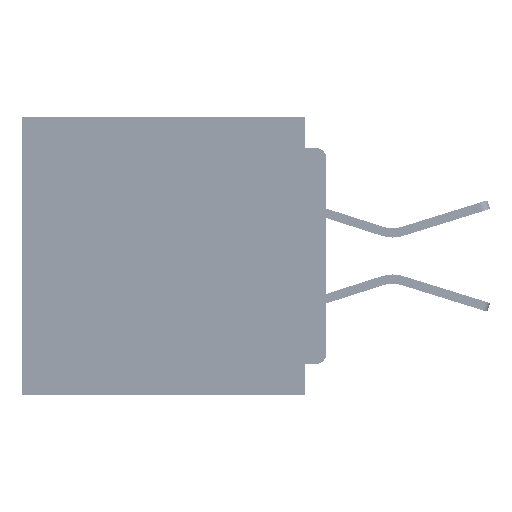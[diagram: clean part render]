
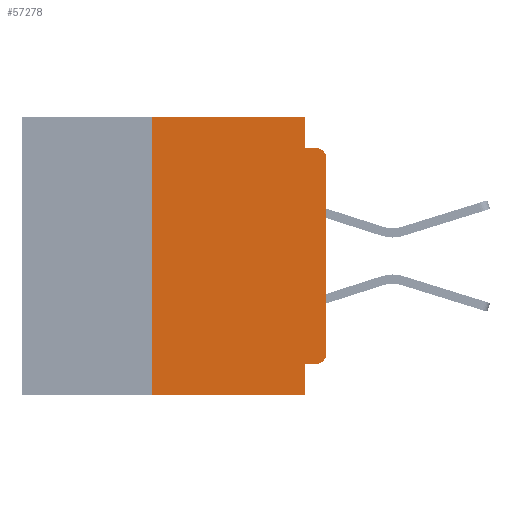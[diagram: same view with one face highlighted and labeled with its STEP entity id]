
A CAD part, left-side view. The second image highlights one B-rep face of the part: STEP entity #57278.
In plain terms, the highlighted planar face has unit normal (-1, 0, 0).
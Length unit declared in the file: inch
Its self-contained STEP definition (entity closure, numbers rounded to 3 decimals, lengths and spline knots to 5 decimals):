
#643 = ORIENTED_EDGE ( 'NONE', *, *, #56176, .F. ) ;
#1257 = AXIS2_PLACEMENT_3D ( 'NONE', #48206, #16533, #53520 ) ;
#1712 = EDGE_CURVE ( 'NONE', #65344, #35225, #22927, .T. ) ;
#2363 = VECTOR ( 'NONE', #48144, 39.37008 ) ;
#2925 = VERTEX_POINT ( 'NONE', #28663 ) ;
#3128 = CARTESIAN_POINT ( 'NONE',  ( 0., 0., -0.045 ) ) ;
#3157 = CIRCLE ( 'NONE', #41771, 0.015 ) ;
#3234 = CARTESIAN_POINT ( 'NONE',  ( 0., 0.015, -0.355 ) ) ;
#4686 = LINE ( 'NONE', #14722, #60964 ) ;
#6895 = DIRECTION ( 'NONE',  ( 0., -1., 0. ) ) ;
#7356 = LINE ( 'NONE', #35289, #61928 ) ;
#8021 = DIRECTION ( 'NONE',  ( 0., 0., 1. ) ) ;
#8457 = ORIENTED_EDGE ( 'NONE', *, *, #18073, .T. ) ;
#8609 = ORIENTED_EDGE ( 'NONE', *, *, #56729, .F. ) ;
#11054 = EDGE_CURVE ( 'NONE', #37208, #35153, #3157, .T. ) ;
#11843 = VECTOR ( 'NONE', #43680, 39.37008 ) ;
#12291 = DIRECTION ( 'NONE',  ( 0., 0., -1. ) ) ;
#12355 = DIRECTION ( 'NONE',  ( -1., 0., 0. ) ) ;
#12444 = CARTESIAN_POINT ( 'NONE',  ( 0., 0.015, -0.06 ) ) ;
#12999 = ORIENTED_EDGE ( 'NONE', *, *, #53912, .F. ) ;
#13603 = CARTESIAN_POINT ( 'NONE',  ( 0., 0.031, -0.4 ) ) ;
#14722 = CARTESIAN_POINT ( 'NONE',  ( 0., 0., -0.355 ) ) ;
#15848 = LINE ( 'NONE', #42786, #17516 ) ;
#16228 = ORIENTED_EDGE ( 'NONE', *, *, #58459, .T. ) ;
#16316 = VERTEX_POINT ( 'NONE', #13603 ) ;
#16397 = DIRECTION ( 'NONE',  ( 0., -1., 0. ) ) ;
#16533 = DIRECTION ( 'NONE',  ( 1., 0., 0. ) ) ;
#17516 = VECTOR ( 'NONE', #16397, 39.37008 ) ;
#18073 = EDGE_CURVE ( 'NONE', #35153, #65344, #24891, .T. ) ;
#20800 = DIRECTION ( 'NONE',  ( -1., 0., 0. ) ) ;
#20991 = EDGE_CURVE ( 'NONE', #27909, #35225, #48435, .T. ) ;
#22014 = VERTEX_POINT ( 'NONE', #34155 ) ;
#22927 = CIRCLE ( 'NONE', #64761, 0.015 ) ;
#23012 = CARTESIAN_POINT ( 'NONE',  ( 0., 0.031, 0. ) ) ;
#23537 = EDGE_CURVE ( 'NONE', #37208, #55369, #4686, .T. ) ;
#24891 = LINE ( 'NONE', #55711, #49696 ) ;
#26288 = CARTESIAN_POINT ( 'NONE',  ( 0., 0.031, -0.045 ) ) ;
#26915 = CARTESIAN_POINT ( 'NONE',  ( 0., 0.031, -0.4 ) ) ;
#27717 = CARTESIAN_POINT ( 'NONE',  ( 0., 0.25, -0.4 ) ) ;
#27869 = ORIENTED_EDGE ( 'NONE', *, *, #23537, .F. ) ;
#27909 = VERTEX_POINT ( 'NONE', #26288 ) ;
#28663 = CARTESIAN_POINT ( 'NONE',  ( 0., 0.25, -0.4 ) ) ;
#32731 = VECTOR ( 'NONE', #61667, 39.37008 ) ;
#34155 = CARTESIAN_POINT ( 'NONE',  ( 0., 0.25, 0. ) ) ;
#35068 = CARTESIAN_POINT ( 'NONE',  ( 0., 0., -0.34 ) ) ;
#35153 = VERTEX_POINT ( 'NONE', #35068 ) ;
#35225 = VERTEX_POINT ( 'NONE', #62008 ) ;
#35289 = CARTESIAN_POINT ( 'NONE',  ( 0., 0.031, 0. ) ) ;
#35664 = ORIENTED_EDGE ( 'NONE', *, *, #20991, .F. ) ;
#37208 = VERTEX_POINT ( 'NONE', #3234 ) ;
#41677 = LINE ( 'NONE', #27717, #11843 ) ;
#41771 = AXIS2_PLACEMENT_3D ( 'NONE', #52461, #20800, #57744 ) ;
#42786 = CARTESIAN_POINT ( 'NONE',  ( 0., 0.437, -0.4 ) ) ;
#42915 = PLANE ( 'NONE',  #1257 ) ;
#43075 = LINE ( 'NONE', #26915, #2363 ) ;
#43680 = DIRECTION ( 'NONE',  ( 0., 0., 1. ) ) ;
#44746 = ORIENTED_EDGE ( 'NONE', *, *, #11054, .T. ) ;
#45253 = ORIENTED_EDGE ( 'NONE', *, *, #1712, .T. ) ;
#45923 = DIRECTION ( 'NONE',  ( 0., 0., -1. ) ) ;
#48144 = DIRECTION ( 'NONE',  ( 0., 0., -1. ) ) ;
#48206 = CARTESIAN_POINT ( 'NONE',  ( 0., 0.437, 0. ) ) ;
#48435 = LINE ( 'NONE', #3128, #32731 ) ;
#49696 = VECTOR ( 'NONE', #8021, 39.37008 ) ;
#50216 = CARTESIAN_POINT ( 'NONE',  ( 0., 0., -0.06 ) ) ;
#51744 = DIRECTION ( 'NONE',  ( 0., 1., 0. ) ) ;
#52461 = CARTESIAN_POINT ( 'NONE',  ( 0., 0.015, -0.34 ) ) ;
#52929 = EDGE_CURVE ( 'NONE', #55369, #16316, #43075, .T. ) ;
#53520 = DIRECTION ( 'NONE',  ( 0., 0., -1. ) ) ;
#53912 = EDGE_CURVE ( 'NONE', #63647, #27909, #7356, .T. ) ;
#54583 = CARTESIAN_POINT ( 'NONE',  ( 0., 0.437, 0. ) ) ;
#55369 = VERTEX_POINT ( 'NONE', #68051 ) ;
#55711 = CARTESIAN_POINT ( 'NONE',  ( 0., 0., 0. ) ) ;
#56176 = EDGE_CURVE ( 'NONE', #22014, #63647, #65625, .T. ) ;
#56729 = EDGE_CURVE ( 'NONE', #2925, #22014, #41677, .T. ) ;
#57278 = ADVANCED_FACE ( 'NONE', ( #59670 ), #42915, .F. ) ;
#57744 = DIRECTION ( 'NONE',  ( 0., 0., -1. ) ) ;
#58459 = EDGE_CURVE ( 'NONE', #2925, #16316, #15848, .T. ) ;
#59670 = FACE_OUTER_BOUND ( 'NONE', #60410, .T. ) ;
#60410 = EDGE_LOOP ( 'NONE', ( #8457, #45253, #35664, #12999, #643, #8609, #16228, #62188, #27869, #44746 ) ) ;
#60659 = VECTOR ( 'NONE', #6895, 39.37008 ) ;
#60964 = VECTOR ( 'NONE', #51744, 39.37008 ) ;
#61667 = DIRECTION ( 'NONE',  ( 0., -1., 0. ) ) ;
#61928 = VECTOR ( 'NONE', #45923, 39.37008 ) ;
#62008 = CARTESIAN_POINT ( 'NONE',  ( 0., 0.015, -0.045 ) ) ;
#62188 = ORIENTED_EDGE ( 'NONE', *, *, #52929, .F. ) ;
#63647 = VERTEX_POINT ( 'NONE', #23012 ) ;
#64761 = AXIS2_PLACEMENT_3D ( 'NONE', #12444, #12355, #12291 ) ;
#65344 = VERTEX_POINT ( 'NONE', #50216 ) ;
#65625 = LINE ( 'NONE', #54583, #60659 ) ;
#68051 = CARTESIAN_POINT ( 'NONE',  ( 0., 0.031, -0.355 ) ) ;
